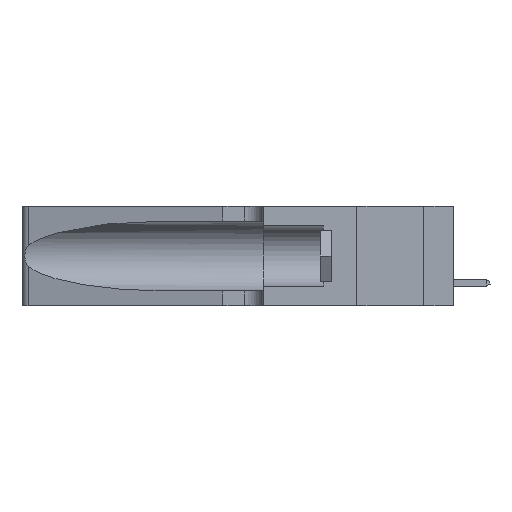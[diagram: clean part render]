
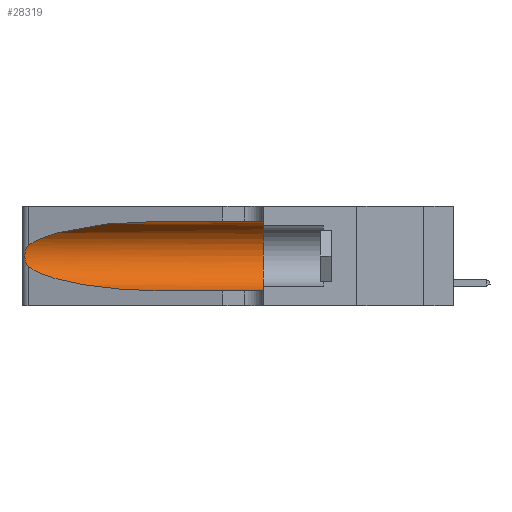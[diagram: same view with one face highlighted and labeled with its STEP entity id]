
A CAD part, left-side view. The second image highlights one B-rep face of the part: STEP entity #28319.
In plain terms, the highlighted cylindrical face has radius 3.308 mm (diameter 6.617 mm), a partial arc.
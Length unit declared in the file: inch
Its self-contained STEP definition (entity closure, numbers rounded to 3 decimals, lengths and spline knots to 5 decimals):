
#185 = AXIS2_PLACEMENT_3D ( 'NONE', #22513, #15337, #818 ) ;
#428 = CARTESIAN_POINT ( 'NONE',  ( 0.25487, 1.22718, 0.22369 ) ) ;
#551 = CARTESIAN_POINT ( 'NONE',  ( 0.25487, 1.22718, 0.14631 ) ) ;
#818 = DIRECTION ( 'NONE',  ( 0., 0., 1. ) ) ;
#841 = EDGE_CURVE ( 'NONE', #18651, #8799, #18194, .T. ) ;
#1336 = DIRECTION ( 'NONE',  ( 0., -1., 0. ) ) ;
#2227 =( BOUNDED_CURVE ( )  B_SPLINE_CURVE ( 3, ( #2472, #6927, #28770, #21717 ),
 .UNSPECIFIED., .F., .F. ) 
 B_SPLINE_CURVE_WITH_KNOTS ( ( 4, 4 ),
 ( 3.44316, 4.71239 ),
 .UNSPECIFIED. ) 
 CURVE ( )  GEOMETRIC_REPRESENTATION_ITEM ( )  RATIONAL_B_SPLINE_CURVE ( ( 1., 0.87, 0.87, 1. ) ) 
 REPRESENTATION_ITEM ( '' )  );
#2472 = CARTESIAN_POINT ( 'NONE',  ( 0.25487, 1.22718, 0.14631 ) ) ;
#2772 = B_SPLINE_CURVE_WITH_KNOTS ( 'NONE', 3,
 ( #428, #2913, #12617, #24617, #17399, #3134, #29712, #29617, #7980, #10408, #29513, #22365, #14860, #551 ),
 .UNSPECIFIED., .F., .F.,
 ( 4, 2, 2, 2, 2, 2, 4 ),
 ( 0., 0.00027, 0.00053, 0.00107, 0.0016, 0.00187, 0.00214 ),
 .UNSPECIFIED. ) ;
#2913 = CARTESIAN_POINT ( 'NONE',  ( 0.25555, 1.22994, 0.2215 ) ) ;
#3134 = CARTESIAN_POINT ( 'NONE',  ( 0.26018, 1.23835, 0.19895 ) ) ;
#3317 = VERTEX_POINT ( 'NONE', #13591 ) ;
#4213 = CARTESIAN_POINT ( 'NONE',  ( 0.25487, 1.22718, 0.14631 ) ) ;
#5544 = EDGE_CURVE ( 'NONE', #14212, #3317, #16777, .T. ) ;
#6024 = CYLINDRICAL_SURFACE ( 'NONE', #24166, 0.13025 ) ;
#6558 = CARTESIAN_POINT ( 'NONE',  ( 0.1305, 0.72297, 0.31525 ) ) ;
#6927 = CARTESIAN_POINT ( 'NONE',  ( 0.2373, 1.15595, 0.08982 ) ) ;
#6970 = CARTESIAN_POINT ( 'NONE',  ( 0.1305, 0.72297, 0.05475 ) ) ;
#7180 = EDGE_CURVE ( 'NONE', #14212, #9383, #18777, .T. ) ;
#7980 = CARTESIAN_POINT ( 'NONE',  ( 0.26017, 1.23833, 0.17102 ) ) ;
#8799 = VERTEX_POINT ( 'NONE', #15324 ) ;
#9383 = VERTEX_POINT ( 'NONE', #20762 ) ;
#10408 = CARTESIAN_POINT ( 'NONE',  ( 0.25856, 1.23593, 0.16098 ) ) ;
#12093 = CARTESIAN_POINT ( 'NONE',  ( 0.25487, 1.22718, 0.22369 ) ) ;
#12499 = VECTOR ( 'NONE', #1336, 39.37008 ) ;
#12617 = CARTESIAN_POINT ( 'NONE',  ( 0.25639, 1.23184, 0.21858 ) ) ;
#12666 = VECTOR ( 'NONE', #27098, 39.37008 ) ;
#12719 = DIRECTION ( 'NONE',  ( 0., 0., -1. ) ) ;
#13433 = EDGE_LOOP ( 'NONE', ( #14898, #20557, #29805, #24165, #18290, #25613 ) ) ;
#13591 = CARTESIAN_POINT ( 'NONE',  ( 0.25487, 1.22718, 0.22369 ) ) ;
#13974 = EDGE_CURVE ( 'NONE', #9383, #8799, #26786, .T. ) ;
#14212 = VERTEX_POINT ( 'NONE', #15241 ) ;
#14781 = FACE_OUTER_BOUND ( 'NONE', #13433, .T. ) ;
#14860 = CARTESIAN_POINT ( 'NONE',  ( 0.25555, 1.22993, 0.14849 ) ) ;
#14898 = ORIENTED_EDGE ( 'NONE', *, *, #5544, .T. ) ;
#15241 = CARTESIAN_POINT ( 'NONE',  ( 0.1305, 0.72297, 0.31525 ) ) ;
#15324 = CARTESIAN_POINT ( 'NONE',  ( 0.1305, 0.35, 0.05475 ) ) ;
#15337 = DIRECTION ( 'NONE',  ( 0., 1., 0. ) ) ;
#16777 =( BOUNDED_CURVE ( )  B_SPLINE_CURVE ( 3, ( #6558, #27711, #31249, #12093 ),
 .UNSPECIFIED., .F., .F. ) 
 B_SPLINE_CURVE_WITH_KNOTS ( ( 4, 4 ),
 ( 1.5708, 2.84003 ),
 .UNSPECIFIED. ) 
 CURVE ( )  GEOMETRIC_REPRESENTATION_ITEM ( )  RATIONAL_B_SPLINE_CURVE ( ( 1., 0.87, 0.87, 1. ) ) 
 REPRESENTATION_ITEM ( '' )  );
#17399 = CARTESIAN_POINT ( 'NONE',  ( 0.25854, 1.2359, 0.20912 ) ) ;
#18194 = LINE ( 'NONE', #30396, #12499 ) ;
#18290 = ORIENTED_EDGE ( 'NONE', *, *, #13974, .F. ) ;
#18651 = VERTEX_POINT ( 'NONE', #6970 ) ;
#18777 = LINE ( 'NONE', #20190, #12666 ) ;
#18785 = EDGE_CURVE ( 'NONE', #23171, #18651, #2227, .T. ) ;
#20190 = CARTESIAN_POINT ( 'NONE',  ( 0.1305, 1.61858, 0.31525 ) ) ;
#20557 = ORIENTED_EDGE ( 'NONE', *, *, #24819, .T. ) ;
#20580 = CARTESIAN_POINT ( 'NONE',  ( 0.1305, 1.61858, 0.185 ) ) ;
#20762 = CARTESIAN_POINT ( 'NONE',  ( 0.1305, 0.35, 0.31525 ) ) ;
#21717 = CARTESIAN_POINT ( 'NONE',  ( 0.1305, 0.72297, 0.05475 ) ) ;
#22365 = CARTESIAN_POINT ( 'NONE',  ( 0.25639, 1.23186, 0.15144 ) ) ;
#22513 = CARTESIAN_POINT ( 'NONE',  ( 0.1305, 0.35, 0.185 ) ) ;
#23171 = VERTEX_POINT ( 'NONE', #4213 ) ;
#24165 = ORIENTED_EDGE ( 'NONE', *, *, #841, .T. ) ;
#24166 = AXIS2_PLACEMENT_3D ( 'NONE', #20580, #29510, #12719 ) ;
#24617 = CARTESIAN_POINT ( 'NONE',  ( 0.25787, 1.23484, 0.2124 ) ) ;
#24819 = EDGE_CURVE ( 'NONE', #3317, #23171, #2772, .T. ) ;
#25613 = ORIENTED_EDGE ( 'NONE', *, *, #7180, .F. ) ;
#26786 = CIRCLE ( 'NONE', #185, 0.13025 ) ;
#27098 = DIRECTION ( 'NONE',  ( 0., -1., 0. ) ) ;
#27711 = CARTESIAN_POINT ( 'NONE',  ( 0.18966, 0.96281, 0.31525 ) ) ;
#28319 = ADVANCED_FACE ( 'NONE', ( #14781 ), #6024, .F. ) ;
#28770 = CARTESIAN_POINT ( 'NONE',  ( 0.18966, 0.96281, 0.05475 ) ) ;
#29510 = DIRECTION ( 'NONE',  ( 0., -1., 0. ) ) ;
#29513 = CARTESIAN_POINT ( 'NONE',  ( 0.25789, 1.23486, 0.15765 ) ) ;
#29617 = CARTESIAN_POINT ( 'NONE',  ( 0.26075, 1.23896, 0.178 ) ) ;
#29712 = CARTESIAN_POINT ( 'NONE',  ( 0.26075, 1.23896, 0.19203 ) ) ;
#29805 = ORIENTED_EDGE ( 'NONE', *, *, #18785, .T. ) ;
#30396 = CARTESIAN_POINT ( 'NONE',  ( 0.1305, 1.61858, 0.05475 ) ) ;
#31249 = CARTESIAN_POINT ( 'NONE',  ( 0.2373, 1.15595, 0.28018 ) ) ;
